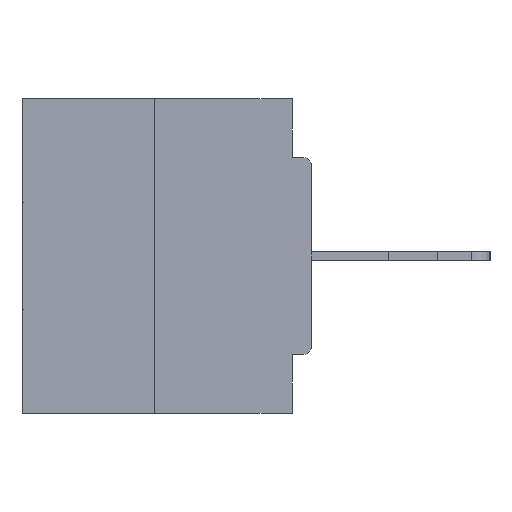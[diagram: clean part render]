
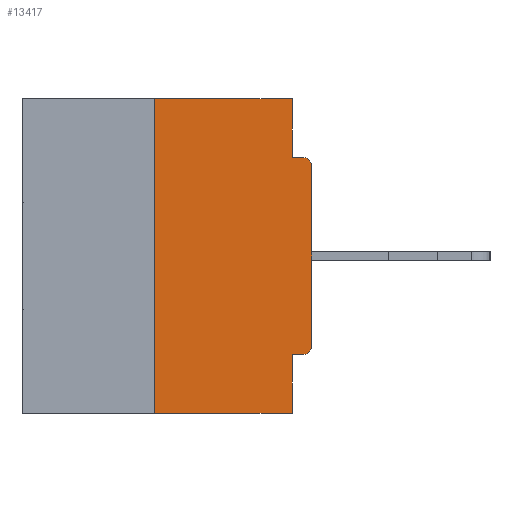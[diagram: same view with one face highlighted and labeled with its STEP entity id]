
A CAD part, left-side view. The second image highlights one B-rep face of the part: STEP entity #13417.
In plain terms, the highlighted planar face has unit normal (-1, 0, 0).
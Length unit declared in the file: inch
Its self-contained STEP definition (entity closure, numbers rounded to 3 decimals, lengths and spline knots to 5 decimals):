
#9 = LINE ( 'NONE', #9536, #28268 ) ;
#498 = LINE ( 'NONE', #33981, #28349 ) ;
#570 = CARTESIAN_POINT ( 'NONE',  ( 0., 0.031, 0. ) ) ;
#580 = VERTEX_POINT ( 'NONE', #11657 ) ;
#613 = CARTESIAN_POINT ( 'NONE',  ( 0., 0.46, 0. ) ) ;
#847 = ORIENTED_EDGE ( 'NONE', *, *, #22721, .F. ) ;
#956 = DIRECTION ( 'NONE',  ( 0., -1., 0. ) ) ;
#1152 = VERTEX_POINT ( 'NONE', #20531 ) ;
#1335 = DIRECTION ( 'NONE',  ( 0., 0., 1. ) ) ;
#2104 = VECTOR ( 'NONE', #4848, 39.37008 ) ;
#2144 = CARTESIAN_POINT ( 'NONE',  ( 0., 0., -0.4065 ) ) ;
#2205 = VERTEX_POINT ( 'NONE', #25774 ) ;
#2631 = EDGE_CURVE ( 'NONE', #26130, #10066, #498, .T. ) ;
#3129 = ORIENTED_EDGE ( 'NONE', *, *, #14263, .F. ) ;
#3154 = VERTEX_POINT ( 'NONE', #6347 ) ;
#3362 = LINE ( 'NONE', #570, #5068 ) ;
#4090 = DIRECTION ( 'NONE',  ( 0., 0., -1. ) ) ;
#4848 = DIRECTION ( 'NONE',  ( 0., 1., 0. ) ) ;
#5068 = VECTOR ( 'NONE', #13506, 39.37008 ) ;
#5102 = CIRCLE ( 'NONE', #24548, 0.015 ) ;
#5210 = CARTESIAN_POINT ( 'NONE',  ( 0., 0.015, -0.4065 ) ) ;
#5713 = ORIENTED_EDGE ( 'NONE', *, *, #18874, .F. ) ;
#5889 = EDGE_CURVE ( 'NONE', #7171, #26130, #5102, .T. ) ;
#6347 = CARTESIAN_POINT ( 'NONE',  ( 0., 0.031, 0. ) ) ;
#6754 = PLANE ( 'NONE',  #10458 ) ;
#6867 = CARTESIAN_POINT ( 'NONE',  ( 0., 0.46, -0.5 ) ) ;
#7171 = VERTEX_POINT ( 'NONE', #5210 ) ;
#8556 = ORIENTED_EDGE ( 'NONE', *, *, #21717, .T. ) ;
#8632 = VERTEX_POINT ( 'NONE', #22282 ) ;
#9294 = DIRECTION ( 'NONE',  ( 0., 0., -1. ) ) ;
#9336 = ORIENTED_EDGE ( 'NONE', *, *, #2631, .T. ) ;
#9420 = DIRECTION ( 'NONE',  ( 0., 0., -1. ) ) ;
#9536 = CARTESIAN_POINT ( 'NONE',  ( 0., 0.25, 0. ) ) ;
#9668 = DIRECTION ( 'NONE',  ( 0., -1., 0. ) ) ;
#10066 = VERTEX_POINT ( 'NONE', #14653 ) ;
#10458 = AXIS2_PLACEMENT_3D ( 'NONE', #30689, #33405, #9420 ) ;
#10789 = LINE ( 'NONE', #6867, #17175 ) ;
#11657 = CARTESIAN_POINT ( 'NONE',  ( 0., 0.25, -0.5 ) ) ;
#12022 = AXIS2_PLACEMENT_3D ( 'NONE', #25068, #25311, #4090 ) ;
#12555 = ORIENTED_EDGE ( 'NONE', *, *, #19754, .F. ) ;
#13417 = ADVANCED_FACE ( 'NONE', ( #31073 ), #6754, .F. ) ;
#13465 = CARTESIAN_POINT ( 'NONE',  ( 0., 0.031, -0.5 ) ) ;
#13506 = DIRECTION ( 'NONE',  ( 0., 0., -1. ) ) ;
#13721 = DIRECTION ( 'NONE',  ( 0., -1., 0. ) ) ;
#14263 = EDGE_CURVE ( 'NONE', #3154, #1152, #3362, .T. ) ;
#14653 = CARTESIAN_POINT ( 'NONE',  ( 0., 0., -0.1085 ) ) ;
#15357 = ORIENTED_EDGE ( 'NONE', *, *, #5889, .T. ) ;
#15836 = EDGE_CURVE ( 'NONE', #580, #20032, #10789, .T. ) ;
#16425 = VECTOR ( 'NONE', #13721, 39.37008 ) ;
#17028 = CARTESIAN_POINT ( 'NONE',  ( 0., 0.031, -0.5 ) ) ;
#17175 = VECTOR ( 'NONE', #9668, 39.37008 ) ;
#17932 = ORIENTED_EDGE ( 'NONE', *, *, #15836, .T. ) ;
#18874 = EDGE_CURVE ( 'NONE', #580, #2205, #9, .T. ) ;
#19754 = EDGE_CURVE ( 'NONE', #1152, #31823, #21903, .T. ) ;
#20032 = VERTEX_POINT ( 'NONE', #13465 ) ;
#20297 = DIRECTION ( 'NONE',  ( 0., 0., 1. ) ) ;
#20364 = EDGE_CURVE ( 'NONE', #2205, #3154, #28593, .T. ) ;
#20531 = CARTESIAN_POINT ( 'NONE',  ( 0., 0.031, -0.0935 ) ) ;
#21231 = DIRECTION ( 'NONE',  ( -1., 0., 0. ) ) ;
#21717 = EDGE_CURVE ( 'NONE', #10066, #31823, #28340, .T. ) ;
#21903 = LINE ( 'NONE', #29911, #16425 ) ;
#22282 = CARTESIAN_POINT ( 'NONE',  ( 0., 0.031, -0.4065 ) ) ;
#22668 = VECTOR ( 'NONE', #9294, 39.37008 ) ;
#22721 = EDGE_CURVE ( 'NONE', #7171, #8632, #31649, .T. ) ;
#23289 = ORIENTED_EDGE ( 'NONE', *, *, #20364, .F. ) ;
#23812 = EDGE_CURVE ( 'NONE', #8632, #20032, #26448, .T. ) ;
#24548 = AXIS2_PLACEMENT_3D ( 'NONE', #32104, #21231, #29728 ) ;
#25068 = CARTESIAN_POINT ( 'NONE',  ( 0., 0.015, -0.1085 ) ) ;
#25311 = DIRECTION ( 'NONE',  ( -1., 0., 0. ) ) ;
#25774 = CARTESIAN_POINT ( 'NONE',  ( 0., 0.25, 0. ) ) ;
#26130 = VERTEX_POINT ( 'NONE', #28170 ) ;
#26448 = LINE ( 'NONE', #17028, #22668 ) ;
#26633 = ORIENTED_EDGE ( 'NONE', *, *, #23812, .F. ) ;
#27003 = EDGE_LOOP ( 'NONE', ( #23289, #5713, #17932, #26633, #847, #15357, #9336, #8556, #12555, #3129 ) ) ;
#27734 = VECTOR ( 'NONE', #956, 39.37008 ) ;
#28170 = CARTESIAN_POINT ( 'NONE',  ( 0., 0., -0.3915 ) ) ;
#28268 = VECTOR ( 'NONE', #1335, 39.37008 ) ;
#28340 = CIRCLE ( 'NONE', #12022, 0.015 ) ;
#28349 = VECTOR ( 'NONE', #20297, 39.37008 ) ;
#28593 = LINE ( 'NONE', #613, #27734 ) ;
#28942 = CARTESIAN_POINT ( 'NONE',  ( 0., 0.015, -0.0935 ) ) ;
#29728 = DIRECTION ( 'NONE',  ( 0., 0., -1. ) ) ;
#29911 = CARTESIAN_POINT ( 'NONE',  ( 0., 0., -0.0935 ) ) ;
#30689 = CARTESIAN_POINT ( 'NONE',  ( 0., 0.46, 0. ) ) ;
#31073 = FACE_OUTER_BOUND ( 'NONE', #27003, .T. ) ;
#31649 = LINE ( 'NONE', #2144, #2104 ) ;
#31823 = VERTEX_POINT ( 'NONE', #28942 ) ;
#32104 = CARTESIAN_POINT ( 'NONE',  ( 0., 0.015, -0.3915 ) ) ;
#33405 = DIRECTION ( 'NONE',  ( 1., 0., 0. ) ) ;
#33981 = CARTESIAN_POINT ( 'NONE',  ( 0., 0., 0. ) ) ;
